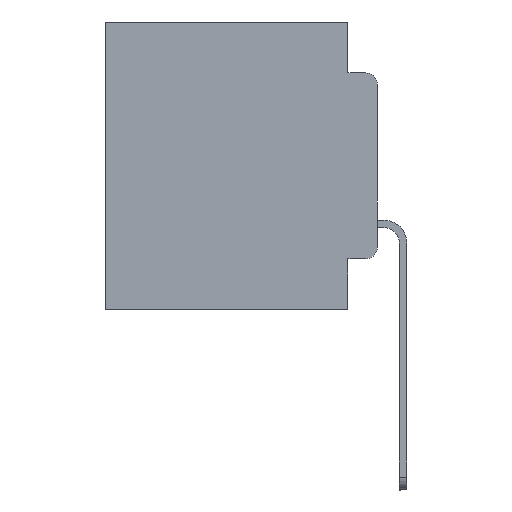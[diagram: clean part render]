
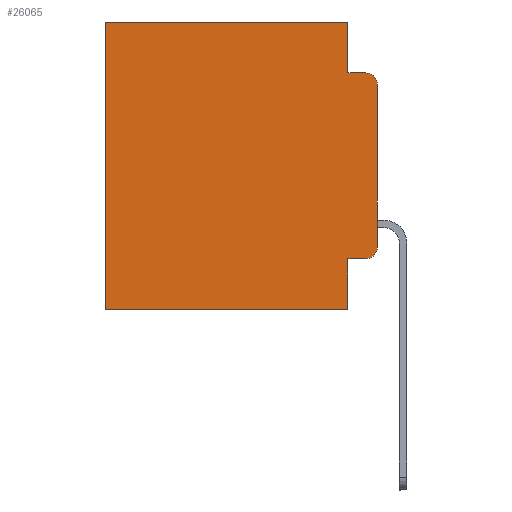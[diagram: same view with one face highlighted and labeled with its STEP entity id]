
A CAD part, left-side view. The second image highlights one B-rep face of the part: STEP entity #26065.
In plain terms, the highlighted planar face has unit normal (-1, 0, 0).
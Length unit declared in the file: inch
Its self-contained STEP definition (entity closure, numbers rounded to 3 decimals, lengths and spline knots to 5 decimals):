
#274 = EDGE_CURVE ( 'NONE', #10150, #22412, #24216, .T. ) ;
#470 = VECTOR ( 'NONE', #21148, 39.37008 ) ;
#1360 = DIRECTION ( 'NONE',  ( -1., 0., 0. ) ) ;
#1713 = LINE ( 'NONE', #14602, #23231 ) ;
#2061 = ORIENTED_EDGE ( 'NONE', *, *, #15942, .T. ) ;
#2138 = DIRECTION ( 'NONE',  ( 0., 1., 0. ) ) ;
#2409 = LINE ( 'NONE', #19753, #14784 ) ;
#2946 = CARTESIAN_POINT ( 'NONE',  ( 0.298, 0.051, -0.0885 ) ) ;
#3567 = DIRECTION ( 'NONE',  ( 0., 0., -1. ) ) ;
#3978 = DIRECTION ( 'NONE',  ( 0., 0., -1. ) ) ;
#4795 = CARTESIAN_POINT ( 'NONE',  ( 0.298, 0.051, -0.5 ) ) ;
#5055 = CIRCLE ( 'NONE', #8035, 0.02 ) ;
#5292 = ORIENTED_EDGE ( 'NONE', *, *, #9198, .F. ) ;
#5590 = EDGE_CURVE ( 'NONE', #12341, #20671, #1713, .T. ) ;
#6579 = VECTOR ( 'NONE', #3978, 39.37008 ) ;
#7077 = EDGE_CURVE ( 'NONE', #20671, #16868, #19843, .T. ) ;
#7507 = AXIS2_PLACEMENT_3D ( 'NONE', #19036, #10401, #16686 ) ;
#8035 = AXIS2_PLACEMENT_3D ( 'NONE', #9754, #16055, #3567 ) ;
#8068 = CARTESIAN_POINT ( 'NONE',  ( 0.298, 0.02, -0.0885 ) ) ;
#8284 = CARTESIAN_POINT ( 'NONE',  ( 0.298, 0.051, -0.4115 ) ) ;
#8387 = ORIENTED_EDGE ( 'NONE', *, *, #7077, .T. ) ;
#8804 = VERTEX_POINT ( 'NONE', #8068 ) ;
#8834 = EDGE_CURVE ( 'NONE', #13787, #21560, #26833, .T. ) ;
#9198 = EDGE_CURVE ( 'NONE', #22412, #16868, #25170, .T. ) ;
#9689 = ORIENTED_EDGE ( 'NONE', *, *, #15338, .F. ) ;
#9754 = CARTESIAN_POINT ( 'NONE',  ( 0.298, 0.02, -0.1085 ) ) ;
#9759 = DIRECTION ( 'NONE',  ( 0., 1., 0. ) ) ;
#9830 = CARTESIAN_POINT ( 'NONE',  ( 0.298, 0.02, -0.3915 ) ) ;
#10150 = VERTEX_POINT ( 'NONE', #12414 ) ;
#10202 = ORIENTED_EDGE ( 'NONE', *, *, #8834, .F. ) ;
#10269 = CIRCLE ( 'NONE', #26206, 0.02 ) ;
#10401 = DIRECTION ( 'NONE',  ( 1., 0., 0. ) ) ;
#10491 = PLANE ( 'NONE',  #7507 ) ;
#10511 = DIRECTION ( 'NONE',  ( 0., -1., 0. ) ) ;
#10966 = LINE ( 'NONE', #2946, #25006 ) ;
#11276 = CARTESIAN_POINT ( 'NONE',  ( 0.298, 0., -0.1085 ) ) ;
#11365 = DIRECTION ( 'NONE',  ( 0., 0., -1. ) ) ;
#11746 = DIRECTION ( 'NONE',  ( 0., 0., -1. ) ) ;
#11872 = ORIENTED_EDGE ( 'NONE', *, *, #14182, .F. ) ;
#12273 = CARTESIAN_POINT ( 'NONE',  ( 0.298, 0., 0. ) ) ;
#12341 = VERTEX_POINT ( 'NONE', #18264 ) ;
#12414 = CARTESIAN_POINT ( 'NONE',  ( 0.298, 0.051, -0.4115 ) ) ;
#13787 = VERTEX_POINT ( 'NONE', #11276 ) ;
#13886 = CARTESIAN_POINT ( 'NONE',  ( 0.298, 0.02, -0.4115 ) ) ;
#14090 = VECTOR ( 'NONE', #9759, 39.37008 ) ;
#14182 = EDGE_CURVE ( 'NONE', #12341, #18340, #2409, .T. ) ;
#14249 = ORIENTED_EDGE ( 'NONE', *, *, #5590, .T. ) ;
#14602 = CARTESIAN_POINT ( 'NONE',  ( 0.298, 0., 0. ) ) ;
#14784 = VECTOR ( 'NONE', #11365, 39.37008 ) ;
#15024 = CARTESIAN_POINT ( 'NONE',  ( 0.298, 0., -0.3915 ) ) ;
#15338 = EDGE_CURVE ( 'NONE', #18340, #8804, #10966, .T. ) ;
#15942 = EDGE_CURVE ( 'NONE', #13787, #8804, #5055, .T. ) ;
#16055 = DIRECTION ( 'NONE',  ( -1., 0., 0. ) ) ;
#16686 = DIRECTION ( 'NONE',  ( 0., 0., -1. ) ) ;
#16868 = VERTEX_POINT ( 'NONE', #26944 ) ;
#16935 = CARTESIAN_POINT ( 'NONE',  ( 0.298, 0.051, -0.0885 ) ) ;
#18078 = CARTESIAN_POINT ( 'NONE',  ( 0.298, 0.473, 0. ) ) ;
#18264 = CARTESIAN_POINT ( 'NONE',  ( 0.298, 0.051, 0. ) ) ;
#18340 = VERTEX_POINT ( 'NONE', #16935 ) ;
#18652 = ORIENTED_EDGE ( 'NONE', *, *, #274, .F. ) ;
#19036 = CARTESIAN_POINT ( 'NONE',  ( 0.298, 0., 0. ) ) ;
#19399 = LINE ( 'NONE', #8284, #470 ) ;
#19753 = CARTESIAN_POINT ( 'NONE',  ( 0.298, 0.051, 0. ) ) ;
#19843 = LINE ( 'NONE', #18078, #20206 ) ;
#20206 = VECTOR ( 'NONE', #20371, 39.37008 ) ;
#20365 = DIRECTION ( 'NONE',  ( 0., 0., -1. ) ) ;
#20371 = DIRECTION ( 'NONE',  ( 0., 0., -1. ) ) ;
#20419 = VERTEX_POINT ( 'NONE', #13886 ) ;
#20660 = VECTOR ( 'NONE', #20365, 39.37008 ) ;
#20671 = VERTEX_POINT ( 'NONE', #26507 ) ;
#21148 = DIRECTION ( 'NONE',  ( 0., -1., 0. ) ) ;
#21560 = VERTEX_POINT ( 'NONE', #15024 ) ;
#22412 = VERTEX_POINT ( 'NONE', #4795 ) ;
#22563 = CARTESIAN_POINT ( 'NONE',  ( 0.298, 0., -0.5 ) ) ;
#22570 = EDGE_LOOP ( 'NONE', ( #10202, #2061, #9689, #11872, #14249, #8387, #5292, #18652, #23780, #25849 ) ) ;
#23231 = VECTOR ( 'NONE', #2138, 39.37008 ) ;
#23780 = ORIENTED_EDGE ( 'NONE', *, *, #25962, .T. ) ;
#24216 = LINE ( 'NONE', #26257, #20660 ) ;
#25006 = VECTOR ( 'NONE', #10511, 39.37008 ) ;
#25170 = LINE ( 'NONE', #22563, #14090 ) ;
#25590 = FACE_OUTER_BOUND ( 'NONE', #22570, .T. ) ;
#25849 = ORIENTED_EDGE ( 'NONE', *, *, #26518, .T. ) ;
#25962 = EDGE_CURVE ( 'NONE', #10150, #20419, #19399, .T. ) ;
#26065 = ADVANCED_FACE ( 'NONE', ( #25590 ), #10491, .F. ) ;
#26206 = AXIS2_PLACEMENT_3D ( 'NONE', #9830, #1360, #11746 ) ;
#26257 = CARTESIAN_POINT ( 'NONE',  ( 0.298, 0.051, 0. ) ) ;
#26507 = CARTESIAN_POINT ( 'NONE',  ( 0.298, 0.473, 0. ) ) ;
#26518 = EDGE_CURVE ( 'NONE', #20419, #21560, #10269, .T. ) ;
#26833 = LINE ( 'NONE', #12273, #6579 ) ;
#26944 = CARTESIAN_POINT ( 'NONE',  ( 0.298, 0.473, -0.5 ) ) ;
